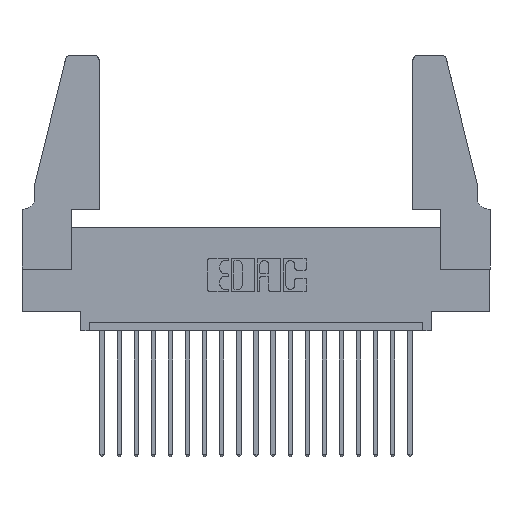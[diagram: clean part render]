
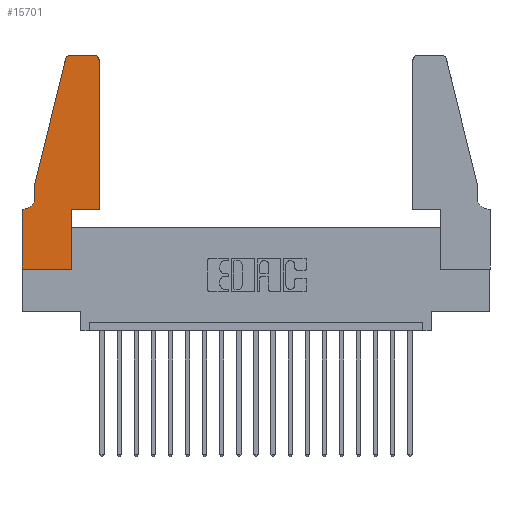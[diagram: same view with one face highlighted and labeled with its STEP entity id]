
A CAD part, top view. The second image highlights one B-rep face of the part: STEP entity #15701.
In plain terms, the highlighted planar face has unit normal (0, 0, 1).
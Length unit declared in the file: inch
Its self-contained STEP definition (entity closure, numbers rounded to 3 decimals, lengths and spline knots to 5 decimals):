
#64 = ORIENTED_EDGE ( 'NONE', *, *, #10850, .T. ) ;
#615 = EDGE_CURVE ( 'NONE', #3954, #16400, #3704, .T. ) ;
#626 = CARTESIAN_POINT ( 'NONE',  ( 0.0055, 0.42, 0.37 ) ) ;
#863 = ORIENTED_EDGE ( 'NONE', *, *, #10293, .T. ) ;
#1508 = EDGE_LOOP ( 'NONE', ( #9243, #64, #16701, #18644, #11775, #12689, #4011, #8138, #18146, #863, #6911, #9743 ) ) ;
#2024 = PLANE ( 'NONE',  #18775 ) ;
#2163 = VERTEX_POINT ( 'NONE', #10785 ) ;
#2510 = VERTEX_POINT ( 'NONE', #14267 ) ;
#2757 = CARTESIAN_POINT ( 'NONE',  ( 0., 0., 0.37 ) ) ;
#3004 = CARTESIAN_POINT ( 'NONE',  ( 0., 0.35, 0.37 ) ) ;
#3019 = AXIS2_PLACEMENT_3D ( 'NONE', #17559, #11575, #11516 ) ;
#3038 = CIRCLE ( 'NONE', #5936, 0.07 ) ;
#3148 = CARTESIAN_POINT ( 'NONE',  ( 0.2865, 0.35, 0.37 ) ) ;
#3275 = CARTESIAN_POINT ( 'NONE',  ( 0.2865, 0., 0.37 ) ) ;
#3413 = DIRECTION ( 'NONE',  ( 1., 0., 0. ) ) ;
#3602 = CARTESIAN_POINT ( 'NONE',  ( 0.0755, 0.5, 0.37 ) ) ;
#3609 = LINE ( 'NONE', #12217, #18370 ) ;
#3704 = LINE ( 'NONE', #18045, #6539 ) ;
#3954 = VERTEX_POINT ( 'NONE', #14486 ) ;
#4011 = ORIENTED_EDGE ( 'NONE', *, *, #6200, .T. ) ;
#4048 = EDGE_CURVE ( 'NONE', #5693, #13899, #5445, .T. ) ;
#4121 = EDGE_CURVE ( 'NONE', #14364, #11208, #12607, .T. ) ;
#4312 = LINE ( 'NONE', #3148, #7140 ) ;
#4341 = EDGE_CURVE ( 'NONE', #11208, #3954, #3038, .T. ) ;
#4526 = DIRECTION ( 'NONE',  ( -1., 0., 0. ) ) ;
#4632 = VECTOR ( 'NONE', #8534, 39.37008 ) ;
#5308 = VECTOR ( 'NONE', #13891, 39.37008 ) ;
#5445 = CIRCLE ( 'NONE', #3019, 0.03 ) ;
#5693 = VERTEX_POINT ( 'NONE', #18894 ) ;
#5936 = AXIS2_PLACEMENT_3D ( 'NONE', #626, #17805, #16407 ) ;
#6200 = EDGE_CURVE ( 'NONE', #16400, #13136, #13843, .T. ) ;
#6539 = VECTOR ( 'NONE', #4526, 39.37008 ) ;
#6911 = ORIENTED_EDGE ( 'NONE', *, *, #13171, .T. ) ;
#6977 = DIRECTION ( 'NONE',  ( 0., 0., 1. ) ) ;
#7011 = CARTESIAN_POINT ( 'NONE',  ( 0.0755, 0.5, 0.37 ) ) ;
#7140 = VECTOR ( 'NONE', #12200, 39.37008 ) ;
#7393 = DIRECTION ( 'NONE',  ( 0., -1., 0. ) ) ;
#7535 = VECTOR ( 'NONE', #11623, 39.37008 ) ;
#8000 = LINE ( 'NONE', #12463, #4632 ) ;
#8138 = ORIENTED_EDGE ( 'NONE', *, *, #8449, .T. ) ;
#8416 = CARTESIAN_POINT ( 'NONE',  ( 0., 0., 0.37 ) ) ;
#8449 = EDGE_CURVE ( 'NONE', #13136, #15718, #14233, .T. ) ;
#8534 = DIRECTION ( 'NONE',  ( 0., 1., 0. ) ) ;
#8585 = DIRECTION ( 'NONE',  ( 1., 0., 0. ) ) ;
#8617 = AXIS2_PLACEMENT_3D ( 'NONE', #17551, #6977, #8585 ) ;
#8844 = FACE_OUTER_BOUND ( 'NONE', #1508, .T. ) ;
#9243 = ORIENTED_EDGE ( 'NONE', *, *, #15409, .T. ) ;
#9247 = CARTESIAN_POINT ( 'NONE',  ( 0.4205, 1.25, 0.37 ) ) ;
#9255 = VECTOR ( 'NONE', #19367, 39.37008 ) ;
#9743 = ORIENTED_EDGE ( 'NONE', *, *, #4048, .T. ) ;
#9836 = VECTOR ( 'NONE', #7393, 39.37008 ) ;
#10293 = EDGE_CURVE ( 'NONE', #13482, #12178, #18227, .T. ) ;
#10389 = VECTOR ( 'NONE', #3413, 39.37008 ) ;
#10785 = CARTESIAN_POINT ( 'NONE',  ( 0.284, 1.25, 0.37 ) ) ;
#10850 = EDGE_CURVE ( 'NONE', #2163, #2510, #17708, .T. ) ;
#10893 = CARTESIAN_POINT ( 'NONE',  ( 0., 0.35, 0.37 ) ) ;
#11061 = LINE ( 'NONE', #15285, #5308 ) ;
#11097 = CARTESIAN_POINT ( 'NONE',  ( 0.4505, 0.35, 0.37 ) ) ;
#11208 = VERTEX_POINT ( 'NONE', #18477 ) ;
#11516 = DIRECTION ( 'NONE',  ( 1., 0., 0. ) ) ;
#11575 = DIRECTION ( 'NONE',  ( 0., 0., 1. ) ) ;
#11623 = DIRECTION ( 'NONE',  ( 1., 0., 0. ) ) ;
#11775 = ORIENTED_EDGE ( 'NONE', *, *, #4341, .T. ) ;
#12095 = DIRECTION ( 'NONE',  ( -1., 0., 0. ) ) ;
#12178 = VERTEX_POINT ( 'NONE', #14627 ) ;
#12200 = DIRECTION ( 'NONE',  ( 0., 1., 0. ) ) ;
#12217 = CARTESIAN_POINT ( 'NONE',  ( 0.2605, 1.25, 0.37 ) ) ;
#12463 = CARTESIAN_POINT ( 'NONE',  ( 0.4505, 0.35, 0.37 ) ) ;
#12607 = LINE ( 'NONE', #7011, #9255 ) ;
#12689 = ORIENTED_EDGE ( 'NONE', *, *, #615, .T. ) ;
#13136 = VERTEX_POINT ( 'NONE', #8416 ) ;
#13171 = EDGE_CURVE ( 'NONE', #12178, #5693, #8000, .T. ) ;
#13482 = VERTEX_POINT ( 'NONE', #17583 ) ;
#13843 = LINE ( 'NONE', #2757, #9836 ) ;
#13891 = DIRECTION ( 'NONE',  ( -0.239, -0.971, 0. ) ) ;
#13899 = VERTEX_POINT ( 'NONE', #9247 ) ;
#13918 = DIRECTION ( 'NONE',  ( 0., 0., 1. ) ) ;
#14233 = LINE ( 'NONE', #16327, #7535 ) ;
#14240 = EDGE_CURVE ( 'NONE', #2510, #14364, #11061, .T. ) ;
#14267 = CARTESIAN_POINT ( 'NONE',  ( 0.25487, 1.22718, 0.37 ) ) ;
#14364 = VERTEX_POINT ( 'NONE', #3602 ) ;
#14486 = CARTESIAN_POINT ( 'NONE',  ( 0.0055, 0.35, 0.37 ) ) ;
#14627 = CARTESIAN_POINT ( 'NONE',  ( 0.4505, 0.35, 0.37 ) ) ;
#15034 = EDGE_CURVE ( 'NONE', #15718, #13482, #4312, .T. ) ;
#15285 = CARTESIAN_POINT ( 'NONE',  ( 0.0755, 0.5, 0.37 ) ) ;
#15409 = EDGE_CURVE ( 'NONE', #13899, #2163, #3609, .T. ) ;
#15701 = ADVANCED_FACE ( 'NONE', ( #8844 ), #2024, .T. ) ;
#15718 = VERTEX_POINT ( 'NONE', #3275 ) ;
#16327 = CARTESIAN_POINT ( 'NONE',  ( 0., 0., 0.37 ) ) ;
#16400 = VERTEX_POINT ( 'NONE', #3004 ) ;
#16407 = DIRECTION ( 'NONE',  ( -1., 0., 0. ) ) ;
#16701 = ORIENTED_EDGE ( 'NONE', *, *, #14240, .T. ) ;
#17551 = CARTESIAN_POINT ( 'NONE',  ( 0.284, 1.22, 0.37 ) ) ;
#17559 = CARTESIAN_POINT ( 'NONE',  ( 0.4205, 1.22, 0.37 ) ) ;
#17583 = CARTESIAN_POINT ( 'NONE',  ( 0.2865, 0.35, 0.37 ) ) ;
#17708 = CIRCLE ( 'NONE', #8617, 0.03 ) ;
#17805 = DIRECTION ( 'NONE',  ( 0., 0., -1. ) ) ;
#18045 = CARTESIAN_POINT ( 'NONE',  ( 0.0755, 0.35, 0.37 ) ) ;
#18146 = ORIENTED_EDGE ( 'NONE', *, *, #15034, .T. ) ;
#18227 = LINE ( 'NONE', #11097, #10389 ) ;
#18370 = VECTOR ( 'NONE', #12095, 39.37008 ) ;
#18477 = CARTESIAN_POINT ( 'NONE',  ( 0.0755, 0.42, 0.37 ) ) ;
#18536 = DIRECTION ( 'NONE',  ( 1., 0., 0. ) ) ;
#18644 = ORIENTED_EDGE ( 'NONE', *, *, #4121, .T. ) ;
#18775 = AXIS2_PLACEMENT_3D ( 'NONE', #10893, #13918, #18536 ) ;
#18894 = CARTESIAN_POINT ( 'NONE',  ( 0.4505, 1.22, 0.37 ) ) ;
#19367 = DIRECTION ( 'NONE',  ( 0., -1., 0. ) ) ;
